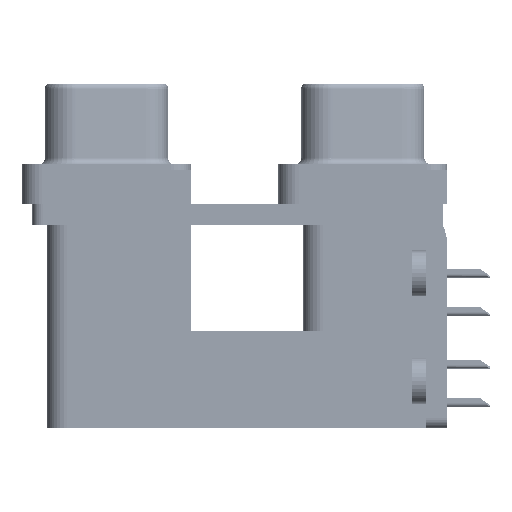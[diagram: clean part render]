
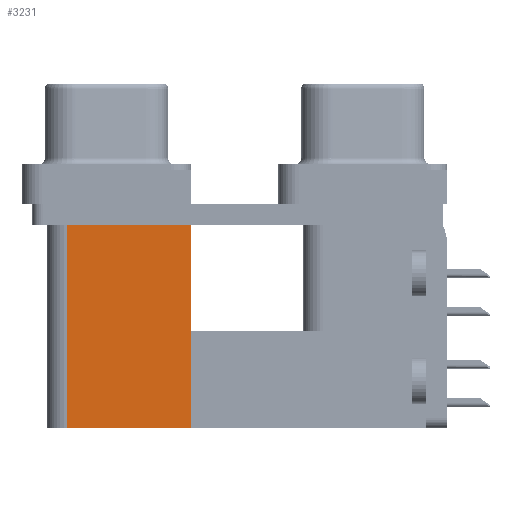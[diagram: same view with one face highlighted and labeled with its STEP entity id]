
A CAD part, left-side view. The second image highlights one B-rep face of the part: STEP entity #3231.
In plain terms, the highlighted planar face has unit normal (-1, 0, 0).
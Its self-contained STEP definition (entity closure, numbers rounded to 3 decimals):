
#1201 = LINE ( 'NONE', #45668, #51221 ) ;
#2662 = VERTEX_POINT ( 'NONE', #35961 ) ;
#3231 = ADVANCED_FACE ( 'NONE', ( #4854 ), #16982, .F. ) ;
#3270 = CARTESIAN_POINT ( 'NONE',  ( 3.79, 21.975, -19.2 ) ) ;
#4725 = CARTESIAN_POINT ( 'NONE',  ( 3.79, 21.975, -19.2 ) ) ;
#4854 = FACE_OUTER_BOUND ( 'NONE', #7998, .T. ) ;
#6061 = ORIENTED_EDGE ( 'NONE', *, *, #49711, .F. ) ;
#6247 = DIRECTION ( 'NONE',  ( 0., 0., 1. ) ) ;
#7998 = EDGE_LOOP ( 'NONE', ( #22673, #16079, #6061, #8785 ) ) ;
#8785 = ORIENTED_EDGE ( 'NONE', *, *, #9567, .T. ) ;
#9501 = LINE ( 'NONE', #47222, #22640 ) ;
#9567 = EDGE_CURVE ( 'NONE', #49285, #2662, #9501, .T. ) ;
#11074 = VECTOR ( 'NONE', #20337, 1000. ) ;
#16079 = ORIENTED_EDGE ( 'NONE', *, *, #44364, .F. ) ;
#16982 = PLANE ( 'NONE',  #46840 ) ;
#18850 = CARTESIAN_POINT ( 'NONE',  ( 3.79, 21.975, -2.5 ) ) ;
#20337 = DIRECTION ( 'NONE',  ( 0., 0., 1. ) ) ;
#21276 = DIRECTION ( 'NONE',  ( 0., 0., -1. ) ) ;
#22640 = VECTOR ( 'NONE', #6247, 1000. ) ;
#22673 = ORIENTED_EDGE ( 'NONE', *, *, #23119, .T. ) ;
#22988 = LINE ( 'NONE', #35944, #31323 ) ;
#23119 = EDGE_CURVE ( 'NONE', #2662, #35993, #1201, .T. ) ;
#23263 = DIRECTION ( 'NONE',  ( 0., 1., 0. ) ) ;
#25185 = DIRECTION ( 'NONE',  ( 0., 1., 0. ) ) ;
#29695 = DIRECTION ( 'NONE',  ( 1., 0., 0. ) ) ;
#31323 = VECTOR ( 'NONE', #23263, 1000. ) ;
#31975 = CARTESIAN_POINT ( 'NONE',  ( 3.79, 12.775, -19.2 ) ) ;
#34240 = CARTESIAN_POINT ( 'NONE',  ( 3.79, 12.775, -19.2 ) ) ;
#34929 = VERTEX_POINT ( 'NONE', #3270 ) ;
#35944 = CARTESIAN_POINT ( 'NONE',  ( 3.79, 12.775, -19.2 ) ) ;
#35961 = CARTESIAN_POINT ( 'NONE',  ( 3.79, 12.775, -2.5 ) ) ;
#35993 = VERTEX_POINT ( 'NONE', #18850 ) ;
#44364 = EDGE_CURVE ( 'NONE', #34929, #35993, #44893, .T. ) ;
#44893 = LINE ( 'NONE', #4725, #11074 ) ;
#45668 = CARTESIAN_POINT ( 'NONE',  ( 3.79, 12.775, -2.5 ) ) ;
#46840 = AXIS2_PLACEMENT_3D ( 'NONE', #34240, #29695, #21276 ) ;
#47222 = CARTESIAN_POINT ( 'NONE',  ( 3.79, 12.775, -19.2 ) ) ;
#49285 = VERTEX_POINT ( 'NONE', #31975 ) ;
#49711 = EDGE_CURVE ( 'NONE', #49285, #34929, #22988, .T. ) ;
#51221 = VECTOR ( 'NONE', #25185, 1000. ) ;
